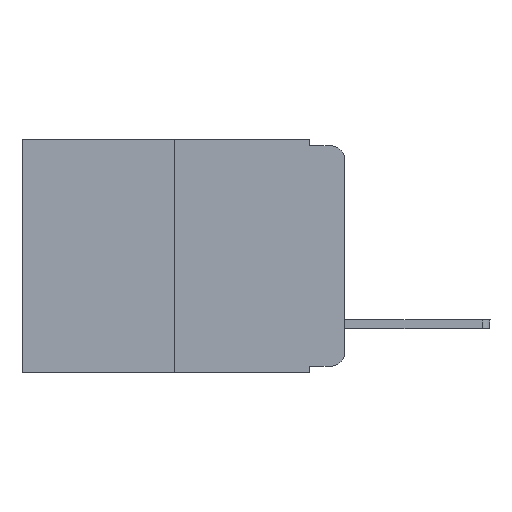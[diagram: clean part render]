
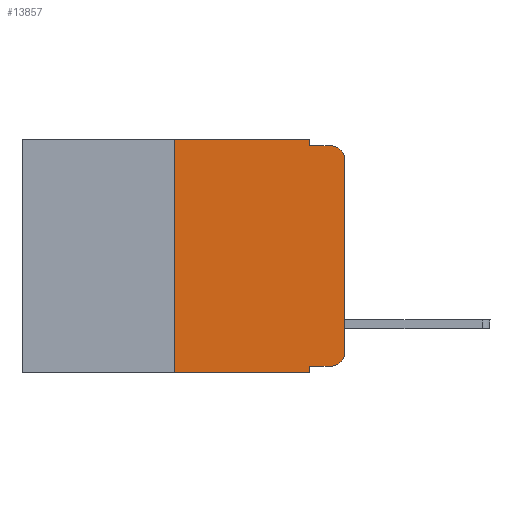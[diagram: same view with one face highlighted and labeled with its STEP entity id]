
A CAD part, left-side view. The second image highlights one B-rep face of the part: STEP entity #13857.
In plain terms, the highlighted planar face has unit normal (-1, 0, 0).
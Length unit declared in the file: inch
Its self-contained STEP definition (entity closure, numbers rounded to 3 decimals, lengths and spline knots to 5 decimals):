
#232 = ORIENTED_EDGE ( 'NONE', *, *, #23416, .T. ) ;
#570 = DIRECTION ( 'NONE',  ( 0., 0., 1. ) ) ;
#690 = DIRECTION ( 'NONE',  ( 0., 0., -1. ) ) ;
#754 = VECTOR ( 'NONE', #21295, 39.37008 ) ;
#812 = DIRECTION ( 'NONE',  ( 0., -1., 0. ) ) ;
#1036 = FACE_OUTER_BOUND ( 'NONE', #20644, .T. ) ;
#1254 = CARTESIAN_POINT ( 'NONE',  ( 0., 0.473, -0.343 ) ) ;
#1459 = ORIENTED_EDGE ( 'NONE', *, *, #19126, .T. ) ;
#1734 = LINE ( 'NONE', #19920, #18607 ) ;
#2241 = VERTEX_POINT ( 'NONE', #16894 ) ;
#2509 = VECTOR ( 'NONE', #2692, 39.37008 ) ;
#2592 = EDGE_CURVE ( 'NONE', #16750, #10340, #8837, .T. ) ;
#2692 = DIRECTION ( 'NONE',  ( 0., 0., -1. ) ) ;
#3336 = CARTESIAN_POINT ( 'NONE',  ( 0., 0.25, -0.343 ) ) ;
#4530 = VECTOR ( 'NONE', #23395, 39.37008 ) ;
#4601 = CARTESIAN_POINT ( 'NONE',  ( 0., 0.473, 0. ) ) ;
#4686 = DIRECTION ( 'NONE',  ( 1., 0., 0. ) ) ;
#4793 = VERTEX_POINT ( 'NONE', #11030 ) ;
#5272 = DIRECTION ( 'NONE',  ( 0., -1., 0. ) ) ;
#5529 = CARTESIAN_POINT ( 'NONE',  ( 0., 0.051, -0.01 ) ) ;
#5568 = VECTOR ( 'NONE', #812, 39.37008 ) ;
#5826 = CARTESIAN_POINT ( 'NONE',  ( 0., 0.051, 0. ) ) ;
#5952 = CARTESIAN_POINT ( 'NONE',  ( 0., 0.051, -0.343 ) ) ;
#6280 = CARTESIAN_POINT ( 'NONE',  ( 0., 0., 0. ) ) ;
#6325 = CARTESIAN_POINT ( 'NONE',  ( 0., 0.02, -0.03 ) ) ;
#6785 = VERTEX_POINT ( 'NONE', #11303 ) ;
#7333 = CIRCLE ( 'NONE', #15798, 0.02 ) ;
#7942 = ORIENTED_EDGE ( 'NONE', *, *, #12894, .F. ) ;
#8039 = ORIENTED_EDGE ( 'NONE', *, *, #22082, .F. ) ;
#8545 = ORIENTED_EDGE ( 'NONE', *, *, #9845, .F. ) ;
#8837 = LINE ( 'NONE', #15821, #2509 ) ;
#9845 = EDGE_CURVE ( 'NONE', #18509, #16750, #10384, .T. ) ;
#10279 = DIRECTION ( 'NONE',  ( -1., 0., 0. ) ) ;
#10340 = VERTEX_POINT ( 'NONE', #21693 ) ;
#10384 = LINE ( 'NONE', #23888, #5568 ) ;
#10392 = PLANE ( 'NONE',  #16014 ) ;
#10468 = VERTEX_POINT ( 'NONE', #18173 ) ;
#10757 = CARTESIAN_POINT ( 'NONE',  ( 0., 0.02, -0.313 ) ) ;
#11015 = AXIS2_PLACEMENT_3D ( 'NONE', #10757, #18157, #20257 ) ;
#11030 = CARTESIAN_POINT ( 'NONE',  ( 0., 0.051, -0.333 ) ) ;
#11134 = VECTOR ( 'NONE', #13775, 39.37008 ) ;
#11303 = CARTESIAN_POINT ( 'NONE',  ( 0., 0.02, -0.333 ) ) ;
#12597 = LINE ( 'NONE', #6280, #24318 ) ;
#12894 = EDGE_CURVE ( 'NONE', #14865, #18509, #1734, .T. ) ;
#12961 = EDGE_CURVE ( 'NONE', #6785, #2241, #21618, .T. ) ;
#13269 = LINE ( 'NONE', #1254, #13853 ) ;
#13471 = LINE ( 'NONE', #5826, #754 ) ;
#13479 = CARTESIAN_POINT ( 'NONE',  ( 0., 0.02, -0.01 ) ) ;
#13775 = DIRECTION ( 'NONE',  ( 0., -1., 0. ) ) ;
#13853 = VECTOR ( 'NONE', #5272, 39.37008 ) ;
#13857 = ADVANCED_FACE ( 'NONE', ( #1036 ), #10392, .F. ) ;
#14865 = VERTEX_POINT ( 'NONE', #3336 ) ;
#15627 = ORIENTED_EDGE ( 'NONE', *, *, #2592, .F. ) ;
#15798 = AXIS2_PLACEMENT_3D ( 'NONE', #6325, #10279, #23740 ) ;
#15821 = CARTESIAN_POINT ( 'NONE',  ( 0., 0.051, 0. ) ) ;
#16014 = AXIS2_PLACEMENT_3D ( 'NONE', #4601, #4686, #690 ) ;
#16750 = VERTEX_POINT ( 'NONE', #23711 ) ;
#16894 = CARTESIAN_POINT ( 'NONE',  ( 0., 0., -0.313 ) ) ;
#16914 = LINE ( 'NONE', #21501, #4530 ) ;
#17360 = VERTEX_POINT ( 'NONE', #5952 ) ;
#18157 = DIRECTION ( 'NONE',  ( -1., 0., 0. ) ) ;
#18173 = CARTESIAN_POINT ( 'NONE',  ( 0., 0., -0.03 ) ) ;
#18509 = VERTEX_POINT ( 'NONE', #23654 ) ;
#18577 = ORIENTED_EDGE ( 'NONE', *, *, #19728, .F. ) ;
#18607 = VECTOR ( 'NONE', #570, 39.37008 ) ;
#19126 = EDGE_CURVE ( 'NONE', #4793, #6785, #16914, .T. ) ;
#19484 = EDGE_CURVE ( 'NONE', #14865, #17360, #13269, .T. ) ;
#19728 = EDGE_CURVE ( 'NONE', #10340, #24267, #23445, .T. ) ;
#19888 = DIRECTION ( 'NONE',  ( 0., 0., 1. ) ) ;
#19920 = CARTESIAN_POINT ( 'NONE',  ( 0., 0.25, 0. ) ) ;
#20257 = DIRECTION ( 'NONE',  ( 0., 0., -1. ) ) ;
#20471 = ORIENTED_EDGE ( 'NONE', *, *, #12961, .T. ) ;
#20556 = ORIENTED_EDGE ( 'NONE', *, *, #19484, .T. ) ;
#20644 = EDGE_LOOP ( 'NONE', ( #24133, #232, #18577, #15627, #8545, #7942, #20556, #8039, #1459, #20471 ) ) ;
#21208 = EDGE_CURVE ( 'NONE', #2241, #10468, #12597, .T. ) ;
#21295 = DIRECTION ( 'NONE',  ( 0., 0., -1. ) ) ;
#21501 = CARTESIAN_POINT ( 'NONE',  ( 0., 0.051, -0.333 ) ) ;
#21618 = CIRCLE ( 'NONE', #11015, 0.02 ) ;
#21693 = CARTESIAN_POINT ( 'NONE',  ( 0., 0.051, -0.01 ) ) ;
#22082 = EDGE_CURVE ( 'NONE', #4793, #17360, #13471, .T. ) ;
#23395 = DIRECTION ( 'NONE',  ( 0., -1., 0. ) ) ;
#23416 = EDGE_CURVE ( 'NONE', #10468, #24267, #7333, .T. ) ;
#23445 = LINE ( 'NONE', #5529, #11134 ) ;
#23654 = CARTESIAN_POINT ( 'NONE',  ( 0., 0.25, 0. ) ) ;
#23711 = CARTESIAN_POINT ( 'NONE',  ( 0., 0.051, 0. ) ) ;
#23740 = DIRECTION ( 'NONE',  ( 0., 0., -1. ) ) ;
#23888 = CARTESIAN_POINT ( 'NONE',  ( 0., 0.473, 0. ) ) ;
#24133 = ORIENTED_EDGE ( 'NONE', *, *, #21208, .T. ) ;
#24267 = VERTEX_POINT ( 'NONE', #13479 ) ;
#24318 = VECTOR ( 'NONE', #19888, 39.37008 ) ;
